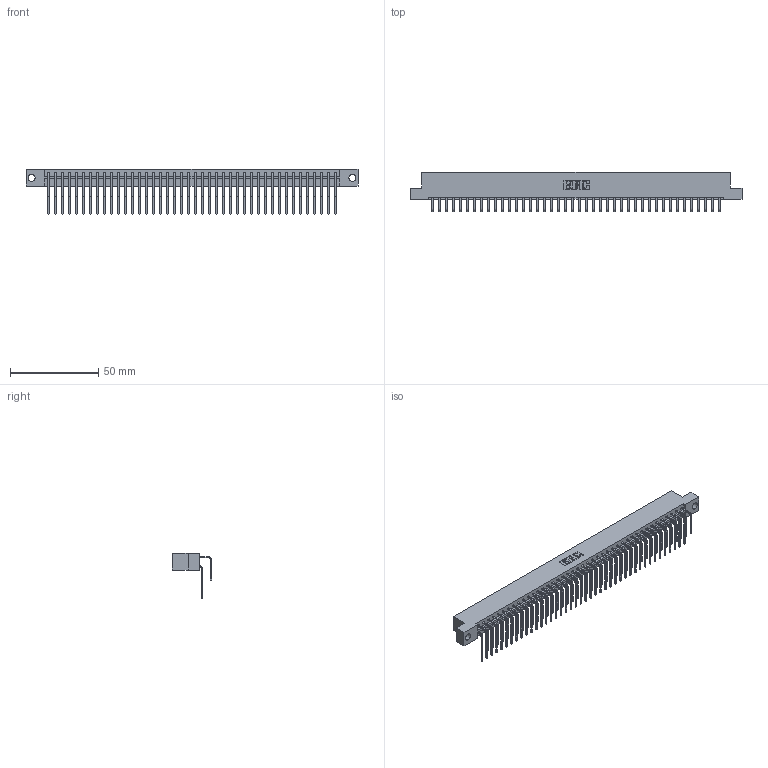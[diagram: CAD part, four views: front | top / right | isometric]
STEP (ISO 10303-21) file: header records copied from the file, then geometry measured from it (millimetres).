
FILE_DESCRIPTION (( 'STEP AP203' ), '1' );
FILE_NAME ('833-084-558-204.STEP', '2020-06-06T02:12:16', ( '' ), ( '' ), 'SwSTEP 2.0', 'SolidWorks 2020', '' );
FILE_SCHEMA (( 'CONFIG_CONTROL_DESIGN' ));
Length unit declared in the file: inch
Products named in the file (4): 833 Part_Flush - .156 Dia - TH; 833-084-558-204; 345-292-001_558 Tail - 2; 345-292-001_558 559 Tail - 1
Assembly tree (85 placements, depth 2):
  833-084-558-204
    833 Part_Flush - .156 Dia - TH
    345-292-001_558 559 Tail - 1  x42
    345-292-001_558 Tail - 2  x42
Bounding box: 187.96 x 22.17 x 25.53 mm (x, y, z)
Volume: 19586.4 mm3; surface area: 25369.1 mm2
Topology: 85 solids, 85 shells, 4650 faces, 13835 edges, 9110 vertices
Faces by surface type: plane 3262, cylinder 1388
Entity records: 28807 total; most frequent: CARTESIAN_POINT 4825, ORIENTED_EDGE 4710, DIRECTION 4103, EDGE_CURVE 2355, LINE 2187, VECTOR 2187, VERTEX_POINT 1566, AXIS2_PLACEMENT_3D 958
